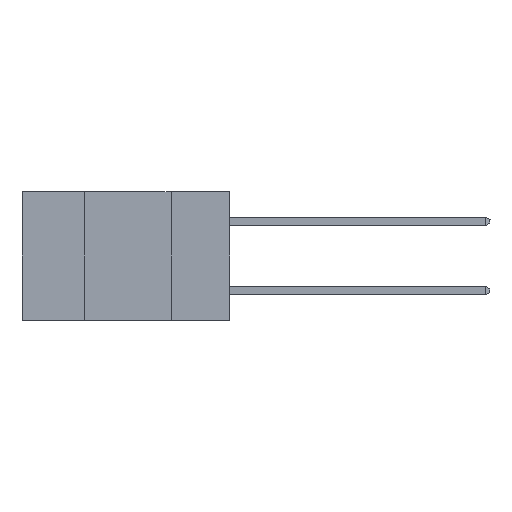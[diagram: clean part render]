
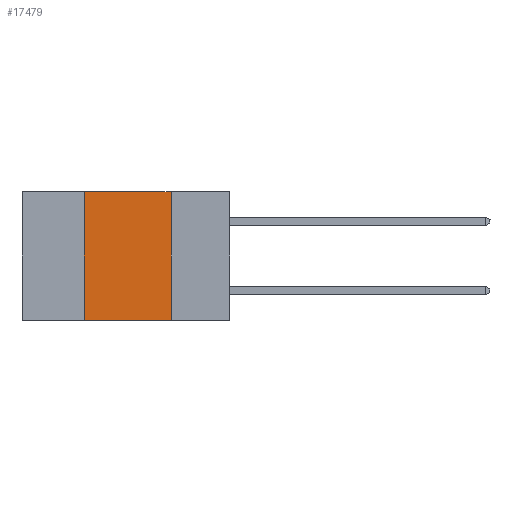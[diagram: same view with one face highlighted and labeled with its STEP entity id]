
A CAD part, left-side view. The second image highlights one B-rep face of the part: STEP entity #17479.
In plain terms, the highlighted planar face has unit normal (-1, 0, 0).
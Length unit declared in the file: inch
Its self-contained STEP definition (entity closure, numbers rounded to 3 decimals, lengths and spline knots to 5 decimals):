
#1606 = EDGE_LOOP ( 'NONE', ( #7753, #1668, #9516, #17313 ) ) ;
#1668 = ORIENTED_EDGE ( 'NONE', *, *, #9891, .F. ) ;
#3488 = LINE ( 'NONE', #12293, #7835 ) ;
#5924 = VERTEX_POINT ( 'NONE', #14142 ) ;
#6772 = VECTOR ( 'NONE', #10359, 39.37008 ) ;
#6855 = DIRECTION ( 'NONE',  ( 0., 0., 1. ) ) ;
#7481 = DIRECTION ( 'NONE',  ( 1., 0., 0. ) ) ;
#7753 = ORIENTED_EDGE ( 'NONE', *, *, #10432, .F. ) ;
#7835 = VECTOR ( 'NONE', #6855, 39.37008 ) ;
#8860 = LINE ( 'NONE', #22049, #10053 ) ;
#9063 = FACE_OUTER_BOUND ( 'NONE', #1606, .T. ) ;
#9516 = ORIENTED_EDGE ( 'NONE', *, *, #18217, .F. ) ;
#9891 = EDGE_CURVE ( 'NONE', #23601, #15110, #8860, .T. ) ;
#10053 = VECTOR ( 'NONE', #10913, 39.37008 ) ;
#10307 = VECTOR ( 'NONE', #21701, 39.37008 ) ;
#10359 = DIRECTION ( 'NONE',  ( 0., 0., -1. ) ) ;
#10432 = EDGE_CURVE ( 'NONE', #15110, #5924, #11792, .T. ) ;
#10913 = DIRECTION ( 'NONE',  ( 0., -1., 0. ) ) ;
#10920 = VERTEX_POINT ( 'NONE', #16294 ) ;
#11270 = DIRECTION ( 'NONE',  ( 0., 0., -1. ) ) ;
#11486 = LINE ( 'NONE', #12214, #10307 ) ;
#11792 = LINE ( 'NONE', #16031, #6772 ) ;
#12214 = CARTESIAN_POINT ( 'NONE',  ( 0., 0.6, -0.37 ) ) ;
#12293 = CARTESIAN_POINT ( 'NONE',  ( 0., 0.42, 0. ) ) ;
#14142 = CARTESIAN_POINT ( 'NONE',  ( 0., 0.17, -0.37 ) ) ;
#15110 = VERTEX_POINT ( 'NONE', #19528 ) ;
#16031 = CARTESIAN_POINT ( 'NONE',  ( 0., 0.17, 0. ) ) ;
#16235 = EDGE_CURVE ( 'NONE', #10920, #5924, #11486, .T. ) ;
#16294 = CARTESIAN_POINT ( 'NONE',  ( 0., 0.42, -0.37 ) ) ;
#17313 = ORIENTED_EDGE ( 'NONE', *, *, #16235, .T. ) ;
#17479 = ADVANCED_FACE ( 'NONE', ( #9063 ), #18725, .F. ) ;
#18217 = EDGE_CURVE ( 'NONE', #10920, #23601, #3488, .T. ) ;
#18414 = CARTESIAN_POINT ( 'NONE',  ( 0., 0.42, 0. ) ) ;
#18725 = PLANE ( 'NONE',  #21106 ) ;
#19528 = CARTESIAN_POINT ( 'NONE',  ( 0., 0.17, 0. ) ) ;
#20672 = CARTESIAN_POINT ( 'NONE',  ( 0., 0.6, 0. ) ) ;
#21106 = AXIS2_PLACEMENT_3D ( 'NONE', #20672, #7481, #11270 ) ;
#21701 = DIRECTION ( 'NONE',  ( 0., -1., 0. ) ) ;
#22049 = CARTESIAN_POINT ( 'NONE',  ( 0., 0.6, 0. ) ) ;
#23601 = VERTEX_POINT ( 'NONE', #18414 ) ;
